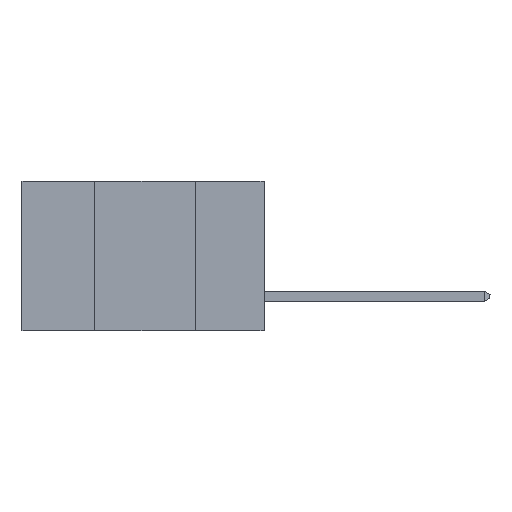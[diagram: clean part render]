
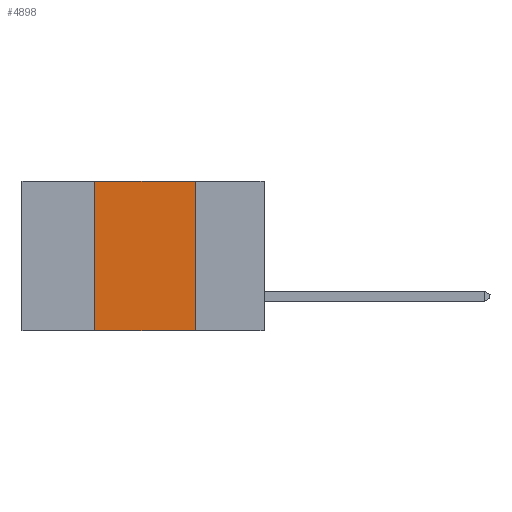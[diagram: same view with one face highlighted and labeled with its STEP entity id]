
A CAD part, left-side view. The second image highlights one B-rep face of the part: STEP entity #4898.
In plain terms, the highlighted planar face has unit normal (-1, 0, 0).
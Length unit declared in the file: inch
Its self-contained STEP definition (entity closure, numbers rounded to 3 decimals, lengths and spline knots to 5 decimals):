
#699 = VERTEX_POINT ( 'NONE', #8475 ) ;
#1541 = ORIENTED_EDGE ( 'NONE', *, *, #22512, .F. ) ;
#3034 = DIRECTION ( 'NONE',  ( 0., -1., 0. ) ) ;
#3101 = ORIENTED_EDGE ( 'NONE', *, *, #23370, .T. ) ;
#3447 = EDGE_CURVE ( 'NONE', #699, #10769, #17200, .T. ) ;
#4284 = EDGE_LOOP ( 'NONE', ( #15522, #1541, #20208, #3101 ) ) ;
#4898 = ADVANCED_FACE ( 'NONE', ( #9221 ), #9512, .F. ) ;
#5558 = VERTEX_POINT ( 'NONE', #22976 ) ;
#5642 = VERTEX_POINT ( 'NONE', #21161 ) ;
#5787 = DIRECTION ( 'NONE',  ( 0., 0., -1. ) ) ;
#7963 = VECTOR ( 'NONE', #16115, 39.37008 ) ;
#8475 = CARTESIAN_POINT ( 'NONE',  ( 0., 0.17, 0. ) ) ;
#9221 = FACE_OUTER_BOUND ( 'NONE', #4284, .T. ) ;
#9512 = PLANE ( 'NONE',  #15275 ) ;
#10419 = DIRECTION ( 'NONE',  ( 0., 0., -1. ) ) ;
#10769 = VERTEX_POINT ( 'NONE', #17725 ) ;
#11124 = VECTOR ( 'NONE', #3034, 39.37008 ) ;
#11494 = EDGE_CURVE ( 'NONE', #5642, #5558, #21322, .T. ) ;
#11695 = VECTOR ( 'NONE', #21284, 39.37008 ) ;
#14003 = CARTESIAN_POINT ( 'NONE',  ( 0., 0.17, 0. ) ) ;
#14900 = DIRECTION ( 'NONE',  ( 1., 0., 0. ) ) ;
#15250 = VECTOR ( 'NONE', #10419, 39.37008 ) ;
#15275 = AXIS2_PLACEMENT_3D ( 'NONE', #22066, #14900, #5787 ) ;
#15522 = ORIENTED_EDGE ( 'NONE', *, *, #3447, .F. ) ;
#15611 = CARTESIAN_POINT ( 'NONE',  ( 0., 0.42, 0. ) ) ;
#16115 = DIRECTION ( 'NONE',  ( 0., -1., 0. ) ) ;
#17200 = LINE ( 'NONE', #14003, #15250 ) ;
#17256 = CARTESIAN_POINT ( 'NONE',  ( 0., 0.6, 0. ) ) ;
#17725 = CARTESIAN_POINT ( 'NONE',  ( 0., 0.17, -0.37 ) ) ;
#20208 = ORIENTED_EDGE ( 'NONE', *, *, #11494, .F. ) ;
#20705 = LINE ( 'NONE', #17256, #11124 ) ;
#21161 = CARTESIAN_POINT ( 'NONE',  ( 0., 0.42, -0.37 ) ) ;
#21284 = DIRECTION ( 'NONE',  ( 0., 0., 1. ) ) ;
#21322 = LINE ( 'NONE', #15611, #11695 ) ;
#21837 = LINE ( 'NONE', #23306, #7963 ) ;
#22066 = CARTESIAN_POINT ( 'NONE',  ( 0., 0.6, 0. ) ) ;
#22512 = EDGE_CURVE ( 'NONE', #5558, #699, #20705, .T. ) ;
#22976 = CARTESIAN_POINT ( 'NONE',  ( 0., 0.42, 0. ) ) ;
#23306 = CARTESIAN_POINT ( 'NONE',  ( 0., 0.6, -0.37 ) ) ;
#23370 = EDGE_CURVE ( 'NONE', #5642, #10769, #21837, .T. ) ;
